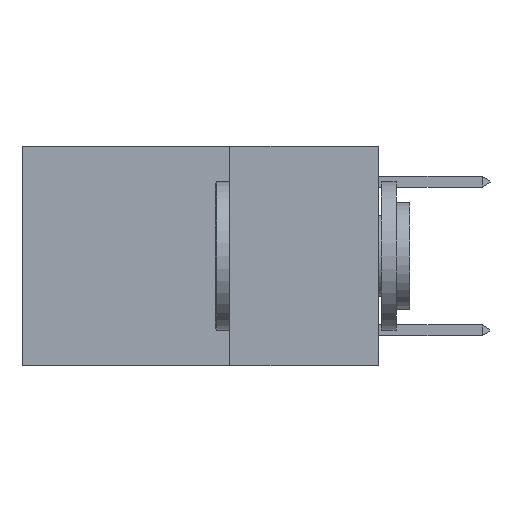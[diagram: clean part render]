
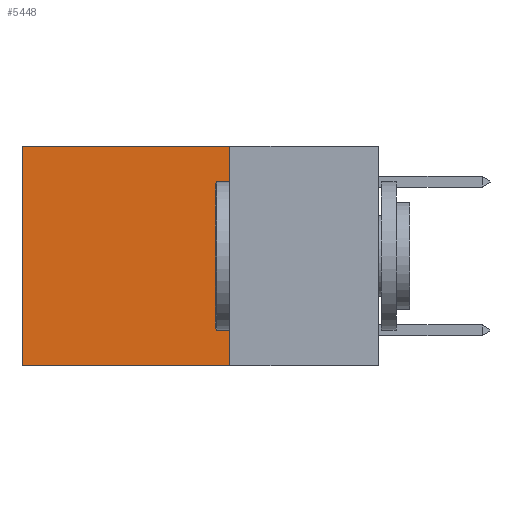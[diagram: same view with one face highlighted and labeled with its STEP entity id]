
A CAD part, left-side view. The second image highlights one B-rep face of the part: STEP entity #5448.
In plain terms, the highlighted planar face has unit normal (-1, 0, 0).
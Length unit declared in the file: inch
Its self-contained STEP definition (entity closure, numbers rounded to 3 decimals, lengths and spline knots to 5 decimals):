
#152 = ORIENTED_EDGE ( 'NONE', *, *, #12017, .T. ) ;
#325 = VECTOR ( 'NONE', #17763, 39.37008 ) ;
#817 = DIRECTION ( 'NONE',  ( 0., 1., 0. ) ) ;
#1151 = EDGE_LOOP ( 'NONE', ( #4406, #6989, #4602, #152 ) ) ;
#1152 = CARTESIAN_POINT ( 'NONE',  ( 0.2625, 0.25, 0. ) ) ;
#2043 = CARTESIAN_POINT ( 'NONE',  ( 0.2625, 0.6, 0. ) ) ;
#2062 = DIRECTION ( 'NONE',  ( 0., 1., 0. ) ) ;
#2381 = LINE ( 'NONE', #11721, #325 ) ;
#3282 = VECTOR ( 'NONE', #4938, 39.37008 ) ;
#4161 = VERTEX_POINT ( 'NONE', #5770 ) ;
#4406 = ORIENTED_EDGE ( 'NONE', *, *, #10710, .T. ) ;
#4602 = ORIENTED_EDGE ( 'NONE', *, *, #15711, .F. ) ;
#4938 = DIRECTION ( 'NONE',  ( 0., 0., -1. ) ) ;
#5131 = LINE ( 'NONE', #10936, #15811 ) ;
#5448 = ADVANCED_FACE ( 'NONE', ( #7012 ), #5590, .F. ) ;
#5590 = PLANE ( 'NONE',  #7732 ) ;
#5770 = CARTESIAN_POINT ( 'NONE',  ( 0.2625, 0.25, -0.37 ) ) ;
#6989 = ORIENTED_EDGE ( 'NONE', *, *, #15967, .F. ) ;
#7012 = FACE_OUTER_BOUND ( 'NONE', #1151, .T. ) ;
#7732 = AXIS2_PLACEMENT_3D ( 'NONE', #12804, #12896, #18593 ) ;
#8563 = VERTEX_POINT ( 'NONE', #10003 ) ;
#9485 = CARTESIAN_POINT ( 'NONE',  ( 0.2625, 0.6, 0. ) ) ;
#10003 = CARTESIAN_POINT ( 'NONE',  ( 0.2625, 0.6, -0.37 ) ) ;
#10710 = EDGE_CURVE ( 'NONE', #17807, #8563, #15080, .T. ) ;
#10936 = CARTESIAN_POINT ( 'NONE',  ( 0.2625, 0.25, -0.37 ) ) ;
#11721 = CARTESIAN_POINT ( 'NONE',  ( 0.2625, 0.25, 0. ) ) ;
#12017 = EDGE_CURVE ( 'NONE', #12734, #17807, #13683, .T. ) ;
#12734 = VERTEX_POINT ( 'NONE', #1152 ) ;
#12804 = CARTESIAN_POINT ( 'NONE',  ( 0.2625, 0.25, 0. ) ) ;
#12896 = DIRECTION ( 'NONE',  ( 1., 0., 0. ) ) ;
#13683 = LINE ( 'NONE', #15286, #14546 ) ;
#14546 = VECTOR ( 'NONE', #2062, 39.37008 ) ;
#15080 = LINE ( 'NONE', #2043, #3282 ) ;
#15286 = CARTESIAN_POINT ( 'NONE',  ( 0.2625, 0.25, 0. ) ) ;
#15711 = EDGE_CURVE ( 'NONE', #12734, #4161, #2381, .T. ) ;
#15811 = VECTOR ( 'NONE', #817, 39.37008 ) ;
#15967 = EDGE_CURVE ( 'NONE', #4161, #8563, #5131, .T. ) ;
#17763 = DIRECTION ( 'NONE',  ( 0., 0., -1. ) ) ;
#17807 = VERTEX_POINT ( 'NONE', #9485 ) ;
#18593 = DIRECTION ( 'NONE',  ( 0., 0., -1. ) ) ;
